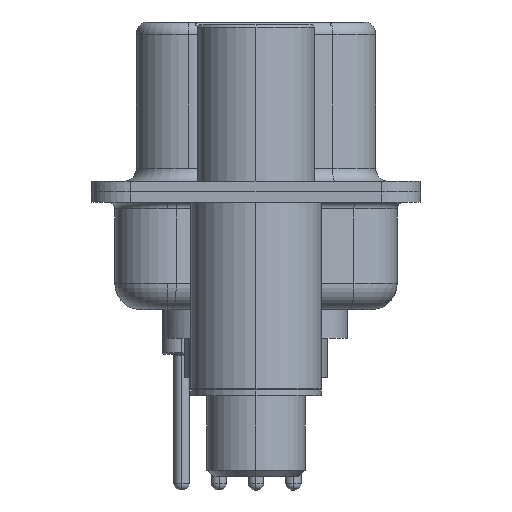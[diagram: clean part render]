
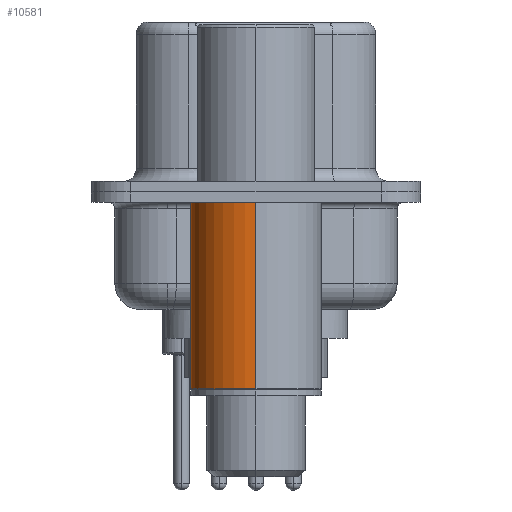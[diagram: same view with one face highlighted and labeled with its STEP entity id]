
A CAD part, left-side view. The second image highlights one B-rep face of the part: STEP entity #10581.
In plain terms, the highlighted cylindrical face has radius 2.5 mm (diameter 5 mm), a partial arc.
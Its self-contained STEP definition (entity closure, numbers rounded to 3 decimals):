
#1107 = CARTESIAN_POINT ( 'NONE',  ( 2.5, 0., -0.4 ) ) ;
#1463 = DIRECTION ( 'NONE',  ( 1., 0., 0. ) ) ;
#1802 = ORIENTED_EDGE ( 'NONE', *, *, #15272, .T. ) ;
#2123 = EDGE_CURVE ( 'NONE', #3878, #6495, #26942, .T. ) ;
#2139 = DIRECTION ( 'NONE',  ( 0., 0., 1. ) ) ;
#3878 = VERTEX_POINT ( 'NONE', #16365 ) ;
#4275 = CYLINDRICAL_SURFACE ( 'NONE', #7111, 2.5 ) ;
#6143 = CIRCLE ( 'NONE', #26582, 2.5 ) ;
#6495 = VERTEX_POINT ( 'NONE', #1107 ) ;
#7019 = ORIENTED_EDGE ( 'NONE', *, *, #2123, .F. ) ;
#7111 = AXIS2_PLACEMENT_3D ( 'NONE', #7702, #20200, #18149 ) ;
#7477 = VERTEX_POINT ( 'NONE', #20682 ) ;
#7702 = CARTESIAN_POINT ( 'NONE',  ( 0., 0., 0.581 ) ) ;
#8526 = LINE ( 'NONE', #21339, #24711 ) ;
#10254 = AXIS2_PLACEMENT_3D ( 'NONE', #26769, #14018, #1463 ) ;
#10581 = ADVANCED_FACE ( 'NONE', ( #26727 ), #4275, .T. ) ;
#10583 = ORIENTED_EDGE ( 'NONE', *, *, #20958, .F. ) ;
#14018 = DIRECTION ( 'NONE',  ( 0., 0., 1. ) ) ;
#14676 = CARTESIAN_POINT ( 'NONE',  ( 0., 0., -7.525 ) ) ;
#15272 = EDGE_CURVE ( 'NONE', #3878, #7477, #6143, .T. ) ;
#16260 = VECTOR ( 'NONE', #25505, 1000. ) ;
#16365 = CARTESIAN_POINT ( 'NONE',  ( 2.5, 0., -7.525 ) ) ;
#16825 = DIRECTION ( 'NONE',  ( 1., 0., 0. ) ) ;
#17475 = ORIENTED_EDGE ( 'NONE', *, *, #26730, .T. ) ;
#18149 = DIRECTION ( 'NONE',  ( 1., 0., 0. ) ) ;
#18257 = VERTEX_POINT ( 'NONE', #23555 ) ;
#18692 = EDGE_LOOP ( 'NONE', ( #1802, #17475, #10583, #7019 ) ) ;
#19220 = DIRECTION ( 'NONE',  ( 0., 0., 1. ) ) ;
#20200 = DIRECTION ( 'NONE',  ( 0., 0., 1. ) ) ;
#20372 = CARTESIAN_POINT ( 'NONE',  ( 2.5, 0., 0.581 ) ) ;
#20682 = CARTESIAN_POINT ( 'NONE',  ( -2.5, 0., -7.525 ) ) ;
#20958 = EDGE_CURVE ( 'NONE', #6495, #18257, #26903, .T. ) ;
#21339 = CARTESIAN_POINT ( 'NONE',  ( -2.5, 0., 0.581 ) ) ;
#23555 = CARTESIAN_POINT ( 'NONE',  ( -2.5, 0., -0.4 ) ) ;
#24711 = VECTOR ( 'NONE', #19220, 1000. ) ;
#25505 = DIRECTION ( 'NONE',  ( 0., 0., 1. ) ) ;
#26582 = AXIS2_PLACEMENT_3D ( 'NONE', #14676, #2139, #16825 ) ;
#26727 = FACE_OUTER_BOUND ( 'NONE', #18692, .T. ) ;
#26730 = EDGE_CURVE ( 'NONE', #7477, #18257, #8526, .T. ) ;
#26769 = CARTESIAN_POINT ( 'NONE',  ( 0., 0., -0.4 ) ) ;
#26903 = CIRCLE ( 'NONE', #10254, 2.5 ) ;
#26942 = LINE ( 'NONE', #20372, #16260 ) ;
